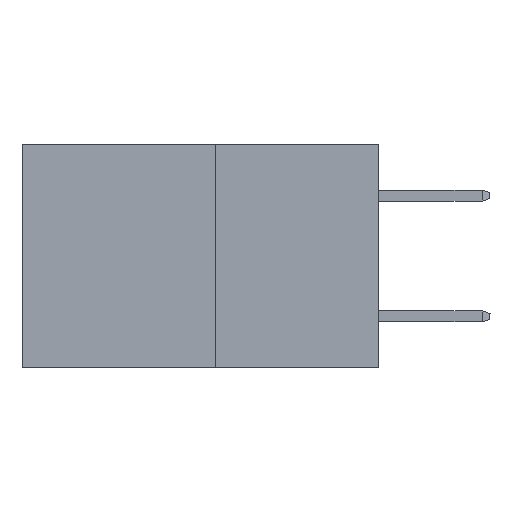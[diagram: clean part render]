
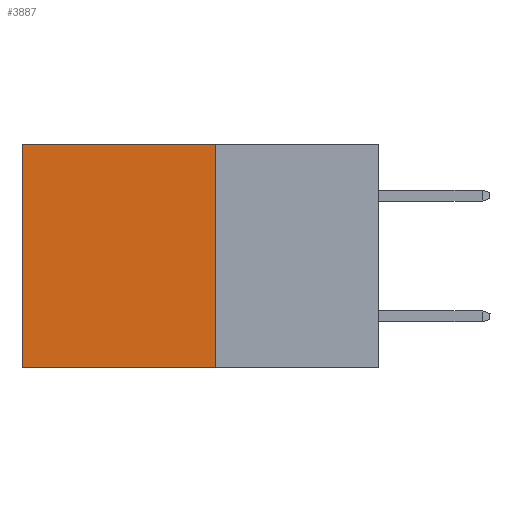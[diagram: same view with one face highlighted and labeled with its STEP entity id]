
A CAD part, left-side view. The second image highlights one B-rep face of the part: STEP entity #3887.
In plain terms, the highlighted planar face has unit normal (-1, 0, 0).
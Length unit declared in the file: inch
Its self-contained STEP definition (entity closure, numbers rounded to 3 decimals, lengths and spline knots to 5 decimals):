
#110 = DIRECTION ( 'NONE',  ( 0., 1., 0. ) ) ;
#278 = VERTEX_POINT ( 'NONE', #2104 ) ;
#2104 = CARTESIAN_POINT ( 'NONE',  ( 0.277, 0.27, -0.37 ) ) ;
#2125 = EDGE_CURVE ( 'NONE', #278, #18109, #15783, .T. ) ;
#2430 = EDGE_CURVE ( 'NONE', #7060, #18109, #3567, .T. ) ;
#2748 = ORIENTED_EDGE ( 'NONE', *, *, #2125, .F. ) ;
#2996 = VECTOR ( 'NONE', #13814, 39.37008 ) ;
#3567 = LINE ( 'NONE', #4912, #2996 ) ;
#3887 = ADVANCED_FACE ( 'NONE', ( #15300 ), #17015, .F. ) ;
#4452 = LINE ( 'NONE', #22386, #18881 ) ;
#4644 = EDGE_CURVE ( 'NONE', #11939, #278, #16120, .T. ) ;
#4912 = CARTESIAN_POINT ( 'NONE',  ( 0.277, 0.59, -0.37 ) ) ;
#5682 = VECTOR ( 'NONE', #23942, 39.37008 ) ;
#6976 = CARTESIAN_POINT ( 'NONE',  ( 0.277, 0.59, 0. ) ) ;
#7060 = VERTEX_POINT ( 'NONE', #6976 ) ;
#7945 = VECTOR ( 'NONE', #22923, 39.37008 ) ;
#10167 = ORIENTED_EDGE ( 'NONE', *, *, #18971, .T. ) ;
#11939 = VERTEX_POINT ( 'NONE', #14811 ) ;
#13814 = DIRECTION ( 'NONE',  ( 0., 0., -1. ) ) ;
#14198 = AXIS2_PLACEMENT_3D ( 'NONE', #17222, #16953, #16887 ) ;
#14811 = CARTESIAN_POINT ( 'NONE',  ( 0.277, 0.27, 0. ) ) ;
#15300 = FACE_OUTER_BOUND ( 'NONE', #21583, .T. ) ;
#15783 = LINE ( 'NONE', #23141, #5682 ) ;
#16120 = LINE ( 'NONE', #23980, #7945 ) ;
#16887 = DIRECTION ( 'NONE',  ( 0., 0., -1. ) ) ;
#16953 = DIRECTION ( 'NONE',  ( 1., 0., 0. ) ) ;
#17015 = PLANE ( 'NONE',  #14198 ) ;
#17217 = ORIENTED_EDGE ( 'NONE', *, *, #2430, .T. ) ;
#17222 = CARTESIAN_POINT ( 'NONE',  ( 0.277, 0.27, -0.37 ) ) ;
#18109 = VERTEX_POINT ( 'NONE', #22265 ) ;
#18881 = VECTOR ( 'NONE', #110, 39.37008 ) ;
#18971 = EDGE_CURVE ( 'NONE', #11939, #7060, #4452, .T. ) ;
#19503 = ORIENTED_EDGE ( 'NONE', *, *, #4644, .F. ) ;
#21583 = EDGE_LOOP ( 'NONE', ( #17217, #2748, #19503, #10167 ) ) ;
#22265 = CARTESIAN_POINT ( 'NONE',  ( 0.277, 0.59, -0.37 ) ) ;
#22386 = CARTESIAN_POINT ( 'NONE',  ( 0.277, 0.27, 0. ) ) ;
#22923 = DIRECTION ( 'NONE',  ( 0., 0., -1. ) ) ;
#23141 = CARTESIAN_POINT ( 'NONE',  ( 0.277, 0.27, -0.37 ) ) ;
#23942 = DIRECTION ( 'NONE',  ( 0., 1., 0. ) ) ;
#23980 = CARTESIAN_POINT ( 'NONE',  ( 0.277, 0.27, -0.37 ) ) ;
